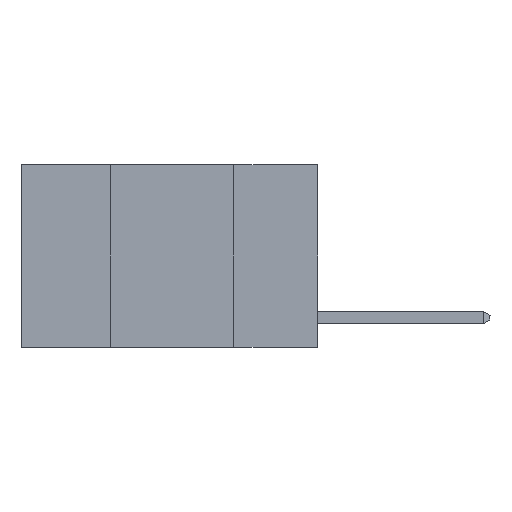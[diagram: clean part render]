
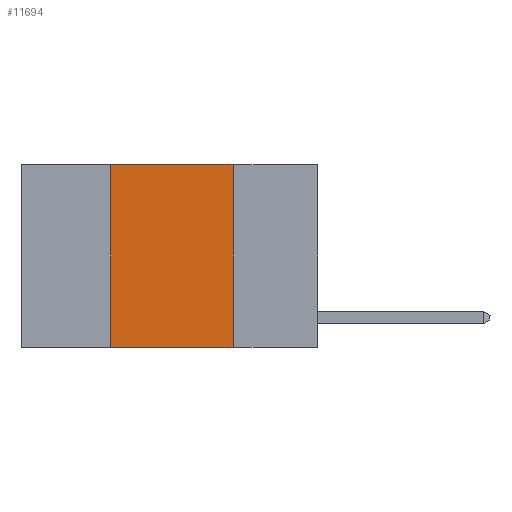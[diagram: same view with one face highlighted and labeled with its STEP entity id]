
A CAD part, left-side view. The second image highlights one B-rep face of the part: STEP entity #11694.
In plain terms, the highlighted planar face has unit normal (-1, 0, 0).
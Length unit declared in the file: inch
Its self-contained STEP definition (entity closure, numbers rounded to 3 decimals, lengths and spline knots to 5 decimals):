
#880 = FACE_OUTER_BOUND ( 'NONE', #10232, .T. ) ;
#1328 = CARTESIAN_POINT ( 'NONE',  ( 0., 0.42, 0. ) ) ;
#1363 = VECTOR ( 'NONE', #12943, 39.37008 ) ;
#1575 = EDGE_CURVE ( 'NONE', #7795, #5016, #6526, .T. ) ;
#1978 = DIRECTION ( 'NONE',  ( 0., 0., 1. ) ) ;
#2419 = EDGE_CURVE ( 'NONE', #3889, #7795, #14903, .T. ) ;
#2492 = DIRECTION ( 'NONE',  ( 0., 0., -1. ) ) ;
#2569 = CARTESIAN_POINT ( 'NONE',  ( 0., 0.17, -0.37 ) ) ;
#2851 = AXIS2_PLACEMENT_3D ( 'NONE', #15451, #15773, #15718 ) ;
#3889 = VERTEX_POINT ( 'NONE', #6608 ) ;
#4126 = CARTESIAN_POINT ( 'NONE',  ( 0., 0.6, -0.37 ) ) ;
#4518 = CARTESIAN_POINT ( 'NONE',  ( 0., 0.17, 0. ) ) ;
#5016 = VERTEX_POINT ( 'NONE', #4518 ) ;
#5082 = DIRECTION ( 'NONE',  ( 0., -1., 0. ) ) ;
#6116 = VECTOR ( 'NONE', #5082, 39.37008 ) ;
#6526 = LINE ( 'NONE', #12495, #6116 ) ;
#6608 = CARTESIAN_POINT ( 'NONE',  ( 0., 0.42, -0.37 ) ) ;
#7795 = VERTEX_POINT ( 'NONE', #1328 ) ;
#8360 = CARTESIAN_POINT ( 'NONE',  ( 0., 0.42, 0. ) ) ;
#8363 = ORIENTED_EDGE ( 'NONE', *, *, #2419, .F. ) ;
#8573 = VECTOR ( 'NONE', #2492, 39.37008 ) ;
#8618 = EDGE_CURVE ( 'NONE', #3889, #9511, #15846, .T. ) ;
#8700 = ORIENTED_EDGE ( 'NONE', *, *, #9528, .F. ) ;
#9511 = VERTEX_POINT ( 'NONE', #2569 ) ;
#9528 = EDGE_CURVE ( 'NONE', #5016, #9511, #13289, .T. ) ;
#10015 = CARTESIAN_POINT ( 'NONE',  ( 0., 0.17, 0. ) ) ;
#10232 = EDGE_LOOP ( 'NONE', ( #8700, #14947, #8363, #12708 ) ) ;
#10396 = PLANE ( 'NONE',  #2851 ) ;
#11694 = ADVANCED_FACE ( 'NONE', ( #880 ), #10396, .F. ) ;
#12495 = CARTESIAN_POINT ( 'NONE',  ( 0., 0.6, 0. ) ) ;
#12708 = ORIENTED_EDGE ( 'NONE', *, *, #8618, .T. ) ;
#12943 = DIRECTION ( 'NONE',  ( 0., -1., 0. ) ) ;
#13289 = LINE ( 'NONE', #10015, #8573 ) ;
#14903 = LINE ( 'NONE', #8360, #15485 ) ;
#14947 = ORIENTED_EDGE ( 'NONE', *, *, #1575, .F. ) ;
#15451 = CARTESIAN_POINT ( 'NONE',  ( 0., 0.6, 0. ) ) ;
#15485 = VECTOR ( 'NONE', #1978, 39.37008 ) ;
#15718 = DIRECTION ( 'NONE',  ( 0., 0., -1. ) ) ;
#15773 = DIRECTION ( 'NONE',  ( 1., 0., 0. ) ) ;
#15846 = LINE ( 'NONE', #4126, #1363 ) ;
